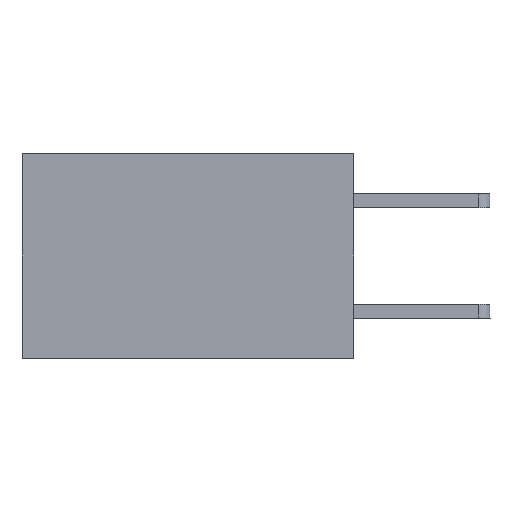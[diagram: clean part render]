
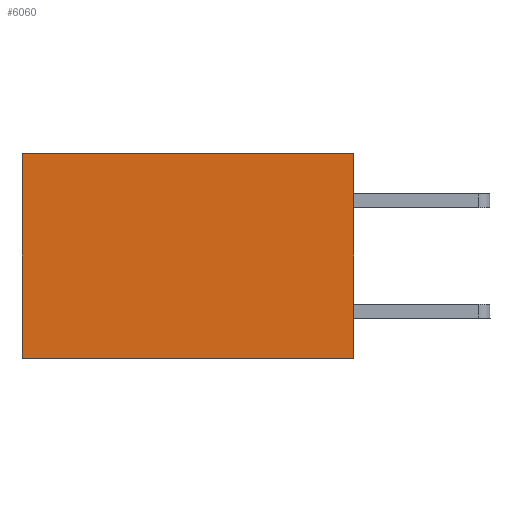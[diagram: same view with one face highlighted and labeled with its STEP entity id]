
A CAD part, left-side view. The second image highlights one B-rep face of the part: STEP entity #6060.
In plain terms, the highlighted planar face has unit normal (-1, 0, 0).
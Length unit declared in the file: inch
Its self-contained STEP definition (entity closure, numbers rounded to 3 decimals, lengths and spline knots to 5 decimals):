
#24 = CARTESIAN_POINT ( 'NONE',  ( 0.2875, 0., 0. ) ) ;
#169 = AXIS2_PLACEMENT_3D ( 'NONE', #9874, #5351, #9751 ) ;
#519 = EDGE_LOOP ( 'NONE', ( #9517, #5431, #8288, #10800 ) ) ;
#966 = CARTESIAN_POINT ( 'NONE',  ( 0.2875, 0., -0.37 ) ) ;
#1037 = VECTOR ( 'NONE', #7223, 39.37008 ) ;
#1374 = CARTESIAN_POINT ( 'NONE',  ( 0.2875, 0., -0.37 ) ) ;
#1486 = DIRECTION ( 'NONE',  ( 0., 1., 0. ) ) ;
#1693 = LINE ( 'NONE', #7675, #9369 ) ;
#2549 = FACE_OUTER_BOUND ( 'NONE', #519, .T. ) ;
#3926 = VECTOR ( 'NONE', #10077, 39.37008 ) ;
#3972 = EDGE_CURVE ( 'NONE', #10647, #8489, #8811, .T. ) ;
#4545 = CARTESIAN_POINT ( 'NONE',  ( 0.2875, 0.6, -0.37 ) ) ;
#4626 = VERTEX_POINT ( 'NONE', #6445 ) ;
#4730 = LINE ( 'NONE', #1374, #9144 ) ;
#4968 = DIRECTION ( 'NONE',  ( 0., 0., -1. ) ) ;
#5351 = DIRECTION ( 'NONE',  ( 1., 0., 0. ) ) ;
#5431 = ORIENTED_EDGE ( 'NONE', *, *, #9575, .F. ) ;
#5814 = EDGE_CURVE ( 'NONE', #4626, #6185, #1693, .T. ) ;
#6060 = ADVANCED_FACE ( 'NONE', ( #2549 ), #8111, .F. ) ;
#6185 = VERTEX_POINT ( 'NONE', #966 ) ;
#6445 = CARTESIAN_POINT ( 'NONE',  ( 0.2875, 0., 0. ) ) ;
#7223 = DIRECTION ( 'NONE',  ( 0., 1., 0. ) ) ;
#7675 = CARTESIAN_POINT ( 'NONE',  ( 0.2875, 0., 0. ) ) ;
#8111 = PLANE ( 'NONE',  #169 ) ;
#8286 = LINE ( 'NONE', #24, #1037 ) ;
#8288 = ORIENTED_EDGE ( 'NONE', *, *, #5814, .F. ) ;
#8489 = VERTEX_POINT ( 'NONE', #4545 ) ;
#8499 = CARTESIAN_POINT ( 'NONE',  ( 0.2875, 0.6, 0. ) ) ;
#8811 = LINE ( 'NONE', #10927, #3926 ) ;
#9144 = VECTOR ( 'NONE', #1486, 39.37008 ) ;
#9369 = VECTOR ( 'NONE', #4968, 39.37008 ) ;
#9517 = ORIENTED_EDGE ( 'NONE', *, *, #3972, .T. ) ;
#9575 = EDGE_CURVE ( 'NONE', #6185, #8489, #4730, .T. ) ;
#9751 = DIRECTION ( 'NONE',  ( 0., 0., -1. ) ) ;
#9874 = CARTESIAN_POINT ( 'NONE',  ( 0.2875, 0., 0. ) ) ;
#10077 = DIRECTION ( 'NONE',  ( 0., 0., -1. ) ) ;
#10647 = VERTEX_POINT ( 'NONE', #8499 ) ;
#10800 = ORIENTED_EDGE ( 'NONE', *, *, #11479, .T. ) ;
#10927 = CARTESIAN_POINT ( 'NONE',  ( 0.2875, 0.6, 0. ) ) ;
#11479 = EDGE_CURVE ( 'NONE', #4626, #10647, #8286, .T. ) ;
